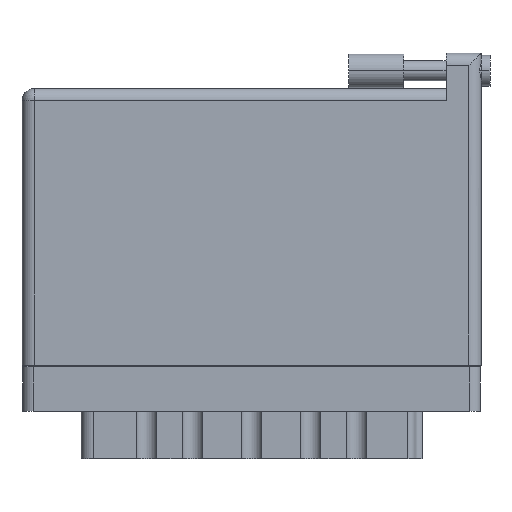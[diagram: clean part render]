
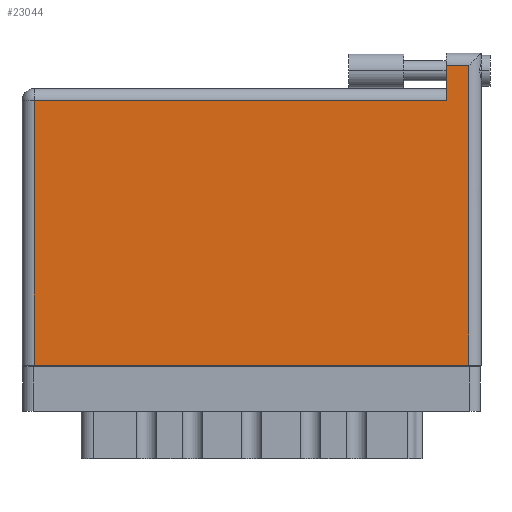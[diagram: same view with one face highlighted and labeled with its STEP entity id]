
A CAD part, front view. The second image highlights one B-rep face of the part: STEP entity #23044.
In plain terms, the highlighted face is planar.
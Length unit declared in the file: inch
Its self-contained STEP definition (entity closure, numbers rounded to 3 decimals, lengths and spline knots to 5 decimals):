
#285 = ORIENTED_EDGE ( 'NONE', *, *, #22527, .T. ) ;
#1897 = CARTESIAN_POINT ( 'NONE',  ( 0., 1.496, 0. ) ) ;
#2462 = CARTESIAN_POINT ( 'NONE',  ( 2.53, 1.696, 0. ) ) ;
#6407 = VECTOR ( 'NONE', #39870, 39.37008 ) ;
#7237 = DIRECTION ( 'NONE',  ( 0., 1., 0. ) ) ;
#9308 = CARTESIAN_POINT ( 'NONE',  ( 2.403, 1.696, 0. ) ) ;
#11730 = VERTEX_POINT ( 'NONE', #35086 ) ;
#12115 = DIRECTION ( 'NONE',  ( -1., 0., 0. ) ) ;
#12593 = LINE ( 'NONE', #48859, #23904 ) ;
#12674 = DIRECTION ( 'NONE',  ( 0., 0., -1. ) ) ;
#12981 = VECTOR ( 'NONE', #28498, 39.37008 ) ;
#14267 = VECTOR ( 'NONE', #33016, 39.37008 ) ;
#16509 = LINE ( 'NONE', #1897, #6407 ) ;
#17789 = LINE ( 'NONE', #36128, #12981 ) ;
#18463 = ORIENTED_EDGE ( 'NONE', *, *, #28922, .T. ) ;
#18897 = VERTEX_POINT ( 'NONE', #37021 ) ;
#19266 = CARTESIAN_POINT ( 'NONE',  ( 2.53, 0., 0. ) ) ;
#20106 = LINE ( 'NONE', #38805, #29146 ) ;
#20214 = EDGE_CURVE ( 'NONE', #33940, #44420, #12593, .T. ) ;
#21038 = CARTESIAN_POINT ( 'NONE',  ( 0., 0., 0. ) ) ;
#22527 = EDGE_CURVE ( 'NONE', #35461, #11730, #16509, .T. ) ;
#23044 = ADVANCED_FACE ( 'NONE', ( #43898 ), #24161, .F. ) ;
#23904 = VECTOR ( 'NONE', #7237, 39.37008 ) ;
#24161 = PLANE ( 'NONE',  #41157 ) ;
#24316 = CARTESIAN_POINT ( 'NONE',  ( 0., 1.566, 0. ) ) ;
#25130 = ORIENTED_EDGE ( 'NONE', *, *, #45589, .T. ) ;
#26806 = LINE ( 'NONE', #21038, #14267 ) ;
#27162 = DIRECTION ( 'NONE',  ( 0., -1., 0. ) ) ;
#27678 = LINE ( 'NONE', #34781, #33020 ) ;
#28498 = DIRECTION ( 'NONE',  ( 0., -1., 0. ) ) ;
#28922 = EDGE_CURVE ( 'NONE', #44420, #32436, #27678, .T. ) ;
#29146 = VECTOR ( 'NONE', #27162, 39.37008 ) ;
#29941 = CARTESIAN_POINT ( 'NONE',  ( 2.403, 1.496, 0. ) ) ;
#32436 = VERTEX_POINT ( 'NONE', #9308 ) ;
#33007 = ORIENTED_EDGE ( 'NONE', *, *, #41015, .T. ) ;
#33016 = DIRECTION ( 'NONE',  ( 1., 0., 0. ) ) ;
#33020 = VECTOR ( 'NONE', #12115, 39.37008 ) ;
#33940 = VERTEX_POINT ( 'NONE', #19266 ) ;
#33976 = EDGE_LOOP ( 'NONE', ( #33007, #41430, #18463, #39284, #285, #25130 ) ) ;
#34781 = CARTESIAN_POINT ( 'NONE',  ( 0., 1.696, 0. ) ) ;
#35086 = CARTESIAN_POINT ( 'NONE',  ( 0.07, 1.496, 0. ) ) ;
#35461 = VERTEX_POINT ( 'NONE', #29941 ) ;
#36128 = CARTESIAN_POINT ( 'NONE',  ( 0.07, 0., 0. ) ) ;
#37021 = CARTESIAN_POINT ( 'NONE',  ( 0.07, 0., 0. ) ) ;
#38805 = CARTESIAN_POINT ( 'NONE',  ( 2.403, 1.766, 0. ) ) ;
#39284 = ORIENTED_EDGE ( 'NONE', *, *, #41389, .T. ) ;
#39870 = DIRECTION ( 'NONE',  ( -1., 0., 0. ) ) ;
#41015 = EDGE_CURVE ( 'NONE', #18897, #33940, #26806, .T. ) ;
#41157 = AXIS2_PLACEMENT_3D ( 'NONE', #24316, #12674, #43471 ) ;
#41389 = EDGE_CURVE ( 'NONE', #32436, #35461, #20106, .T. ) ;
#41430 = ORIENTED_EDGE ( 'NONE', *, *, #20214, .T. ) ;
#43471 = DIRECTION ( 'NONE',  ( -1., 0., 0. ) ) ;
#43898 = FACE_OUTER_BOUND ( 'NONE', #33976, .T. ) ;
#44420 = VERTEX_POINT ( 'NONE', #2462 ) ;
#45589 = EDGE_CURVE ( 'NONE', #11730, #18897, #17789, .T. ) ;
#48859 = CARTESIAN_POINT ( 'NONE',  ( 2.53, 1.766, 0. ) ) ;
